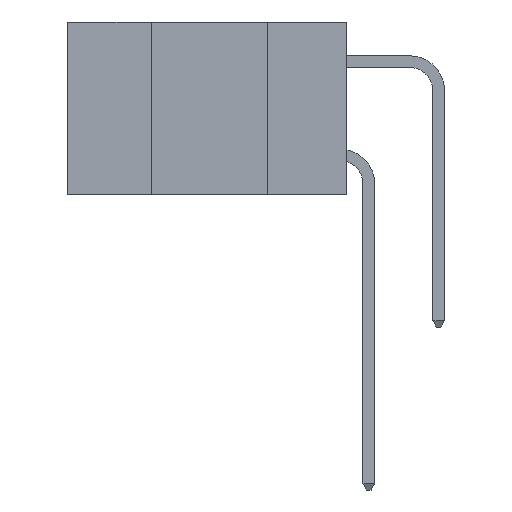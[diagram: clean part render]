
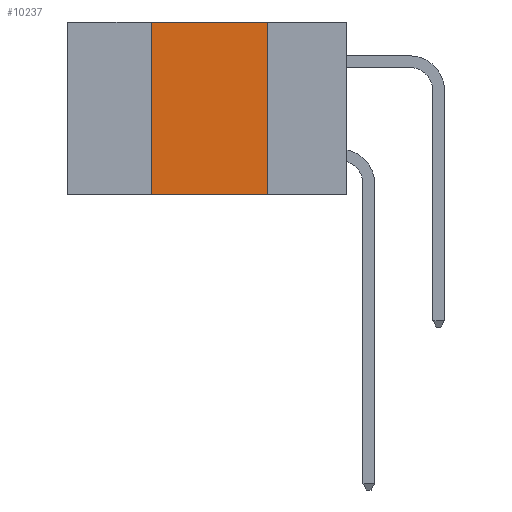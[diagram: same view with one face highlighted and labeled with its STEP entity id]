
A CAD part, left-side view. The second image highlights one B-rep face of the part: STEP entity #10237.
In plain terms, the highlighted planar face has unit normal (-1, 0, 0).
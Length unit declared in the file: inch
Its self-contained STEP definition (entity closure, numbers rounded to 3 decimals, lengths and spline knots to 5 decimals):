
#748 = DIRECTION ( 'NONE',  ( 0., 0., -1. ) ) ;
#1887 = VERTEX_POINT ( 'NONE', #16221 ) ;
#1929 = CARTESIAN_POINT ( 'NONE',  ( 0., 0.42, 0. ) ) ;
#2444 = VECTOR ( 'NONE', #4488, 39.37008 ) ;
#4336 = CARTESIAN_POINT ( 'NONE',  ( 0., 0.42, -0.37 ) ) ;
#4488 = DIRECTION ( 'NONE',  ( 0., -1., 0. ) ) ;
#4881 = ORIENTED_EDGE ( 'NONE', *, *, #24195, .F. ) ;
#4897 = ORIENTED_EDGE ( 'NONE', *, *, #6370, .F. ) ;
#5855 = LINE ( 'NONE', #6506, #2444 ) ;
#6309 = DIRECTION ( 'NONE',  ( 0., 0., 1. ) ) ;
#6370 = EDGE_CURVE ( 'NONE', #16932, #9860, #15151, .T. ) ;
#6506 = CARTESIAN_POINT ( 'NONE',  ( 0., 0.6, -0.37 ) ) ;
#7056 = AXIS2_PLACEMENT_3D ( 'NONE', #20817, #18844, #27716 ) ;
#7240 = EDGE_CURVE ( 'NONE', #16932, #18674, #5855, .T. ) ;
#7435 = CARTESIAN_POINT ( 'NONE',  ( 0., 0.6, 0. ) ) ;
#7470 = ORIENTED_EDGE ( 'NONE', *, *, #7240, .T. ) ;
#9860 = VERTEX_POINT ( 'NONE', #15253 ) ;
#10237 = ADVANCED_FACE ( 'NONE', ( #23065 ), #23375, .F. ) ;
#10740 = VECTOR ( 'NONE', #6309, 39.37008 ) ;
#12880 = VECTOR ( 'NONE', #16144, 39.37008 ) ;
#13102 = CARTESIAN_POINT ( 'NONE',  ( 0., 0.17, 0. ) ) ;
#14077 = ORIENTED_EDGE ( 'NONE', *, *, #17718, .F. ) ;
#14391 = EDGE_LOOP ( 'NONE', ( #14077, #4881, #4897, #7470 ) ) ;
#14875 = VECTOR ( 'NONE', #748, 39.37008 ) ;
#15151 = LINE ( 'NONE', #1929, #10740 ) ;
#15253 = CARTESIAN_POINT ( 'NONE',  ( 0., 0.42, 0. ) ) ;
#16144 = DIRECTION ( 'NONE',  ( 0., -1., 0. ) ) ;
#16221 = CARTESIAN_POINT ( 'NONE',  ( 0., 0.17, 0. ) ) ;
#16248 = LINE ( 'NONE', #13102, #14875 ) ;
#16271 = LINE ( 'NONE', #7435, #12880 ) ;
#16932 = VERTEX_POINT ( 'NONE', #4336 ) ;
#17227 = CARTESIAN_POINT ( 'NONE',  ( 0., 0.17, -0.37 ) ) ;
#17718 = EDGE_CURVE ( 'NONE', #1887, #18674, #16248, .T. ) ;
#18674 = VERTEX_POINT ( 'NONE', #17227 ) ;
#18844 = DIRECTION ( 'NONE',  ( 1., 0., 0. ) ) ;
#20817 = CARTESIAN_POINT ( 'NONE',  ( 0., 0.6, 0. ) ) ;
#23065 = FACE_OUTER_BOUND ( 'NONE', #14391, .T. ) ;
#23375 = PLANE ( 'NONE',  #7056 ) ;
#24195 = EDGE_CURVE ( 'NONE', #9860, #1887, #16271, .T. ) ;
#27716 = DIRECTION ( 'NONE',  ( 0., 0., -1. ) ) ;
